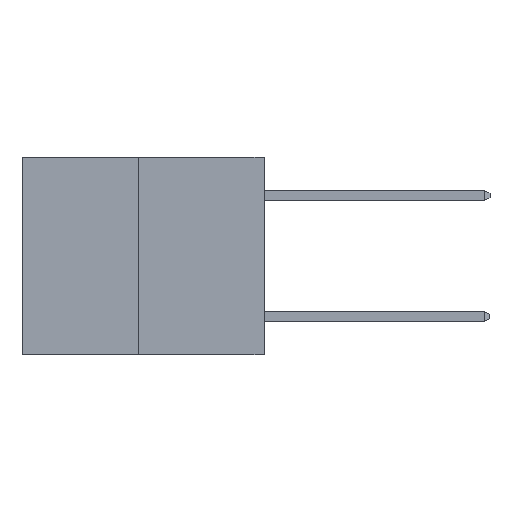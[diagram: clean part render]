
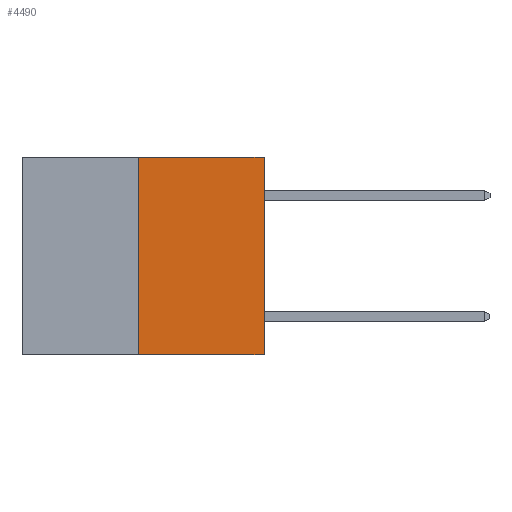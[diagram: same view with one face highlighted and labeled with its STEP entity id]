
A CAD part, left-side view. The second image highlights one B-rep face of the part: STEP entity #4490.
In plain terms, the highlighted planar face has unit normal (-1, 0, 0).
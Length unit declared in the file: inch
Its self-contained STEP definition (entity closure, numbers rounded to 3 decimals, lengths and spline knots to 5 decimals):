
#10 = CARTESIAN_POINT ( 'NONE',  ( 0., 0.312, 0. ) ) ;
#1468 = CARTESIAN_POINT ( 'NONE',  ( 0., 0.312, -0.49 ) ) ;
#1616 = AXIS2_PLACEMENT_3D ( 'NONE', #3553, #11620, #4763 ) ;
#2226 = EDGE_CURVE ( 'NONE', #4291, #10711, #11736, .T. ) ;
#2511 = FACE_OUTER_BOUND ( 'NONE', #12831, .T. ) ;
#3294 = DIRECTION ( 'NONE',  ( 0., -1., 0. ) ) ;
#3553 = CARTESIAN_POINT ( 'NONE',  ( 0., 0.6, 0. ) ) ;
#4060 = ORIENTED_EDGE ( 'NONE', *, *, #2226, .F. ) ;
#4272 = LINE ( 'NONE', #11298, #14699 ) ;
#4291 = VERTEX_POINT ( 'NONE', #10 ) ;
#4409 = ORIENTED_EDGE ( 'NONE', *, *, #6743, .T. ) ;
#4490 = ADVANCED_FACE ( 'NONE', ( #2511 ), #11566, .F. ) ;
#4619 = CARTESIAN_POINT ( 'NONE',  ( 0., 0.6, -0.49 ) ) ;
#4651 = CARTESIAN_POINT ( 'NONE',  ( 0., 0., 0. ) ) ;
#4763 = DIRECTION ( 'NONE',  ( 0., 0., -1. ) ) ;
#6193 = CARTESIAN_POINT ( 'NONE',  ( 0., 0.6, 0. ) ) ;
#6743 = EDGE_CURVE ( 'NONE', #12836, #6949, #12149, .T. ) ;
#6949 = VERTEX_POINT ( 'NONE', #9907 ) ;
#7061 = ORIENTED_EDGE ( 'NONE', *, *, #12987, .F. ) ;
#7307 = VECTOR ( 'NONE', #3294, 39.37008 ) ;
#7547 = VECTOR ( 'NONE', #14172, 39.37008 ) ;
#8642 = LINE ( 'NONE', #1468, #7547 ) ;
#8722 = VECTOR ( 'NONE', #13257, 39.37008 ) ;
#9147 = CARTESIAN_POINT ( 'NONE',  ( 0., 0.312, -0.49 ) ) ;
#9677 = EDGE_CURVE ( 'NONE', #6949, #10711, #4272, .T. ) ;
#9907 = CARTESIAN_POINT ( 'NONE',  ( 0., 0., -0.49 ) ) ;
#10711 = VERTEX_POINT ( 'NONE', #4651 ) ;
#11298 = CARTESIAN_POINT ( 'NONE',  ( 0., 0., 0. ) ) ;
#11566 = PLANE ( 'NONE',  #1616 ) ;
#11620 = DIRECTION ( 'NONE',  ( 1., 0., 0. ) ) ;
#11736 = LINE ( 'NONE', #6193, #8722 ) ;
#12149 = LINE ( 'NONE', #4619, #7307 ) ;
#12449 = ORIENTED_EDGE ( 'NONE', *, *, #9677, .T. ) ;
#12831 = EDGE_LOOP ( 'NONE', ( #7061, #4409, #12449, #4060 ) ) ;
#12836 = VERTEX_POINT ( 'NONE', #9147 ) ;
#12987 = EDGE_CURVE ( 'NONE', #12836, #4291, #8642, .T. ) ;
#13257 = DIRECTION ( 'NONE',  ( 0., -1., 0. ) ) ;
#13596 = DIRECTION ( 'NONE',  ( 0., 0., 1. ) ) ;
#14172 = DIRECTION ( 'NONE',  ( 0., 0., 1. ) ) ;
#14699 = VECTOR ( 'NONE', #13596, 39.37008 ) ;
